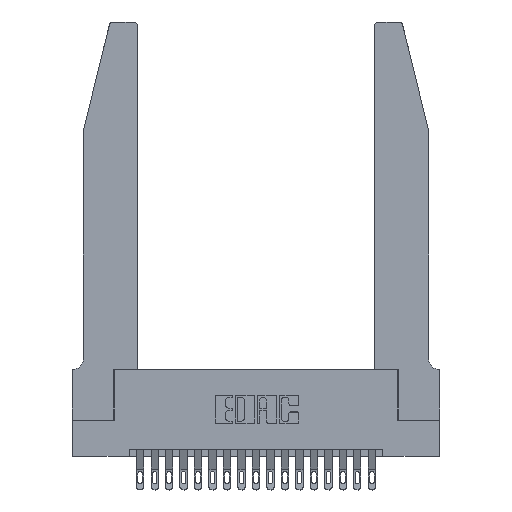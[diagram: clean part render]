
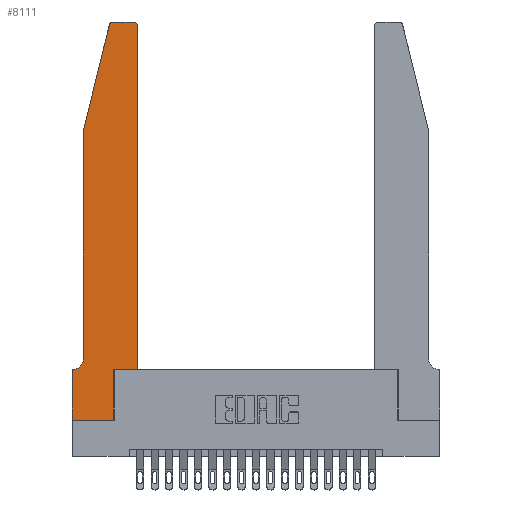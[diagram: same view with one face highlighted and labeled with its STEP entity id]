
A CAD part, top view. The second image highlights one B-rep face of the part: STEP entity #8111.
In plain terms, the highlighted planar face has unit normal (0, 0, 1).
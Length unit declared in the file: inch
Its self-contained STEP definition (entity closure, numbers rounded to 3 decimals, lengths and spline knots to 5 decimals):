
#135 = ORIENTED_EDGE ( 'NONE', *, *, #18145, .T. ) ;
#335 = VERTEX_POINT ( 'NONE', #13361 ) ;
#349 = CARTESIAN_POINT ( 'NONE',  ( 0.4205, 2.72, 0.37 ) ) ;
#358 = DIRECTION ( 'NONE',  ( 0., 0., 1. ) ) ;
#397 = CARTESIAN_POINT ( 'NONE',  ( 0.2605, 2.75, 0.37 ) ) ;
#501 = DIRECTION ( 'NONE',  ( 0., 0., 1. ) ) ;
#661 = DIRECTION ( 'NONE',  ( 1., 0., 0. ) ) ;
#810 = CARTESIAN_POINT ( 'NONE',  ( 0.0755, 0.35, 0.37 ) ) ;
#831 = EDGE_CURVE ( 'NONE', #11296, #10545, #4800, .T. ) ;
#988 = CIRCLE ( 'NONE', #9246, 0.03 ) ;
#994 = EDGE_CURVE ( 'NONE', #17987, #8343, #1332, .T. ) ;
#1332 = LINE ( 'NONE', #8195, #12391 ) ;
#1522 = VERTEX_POINT ( 'NONE', #14327 ) ;
#1997 = VERTEX_POINT ( 'NONE', #9547 ) ;
#2032 = DIRECTION ( 'NONE',  ( 1., 0., 0. ) ) ;
#2087 = DIRECTION ( 'NONE',  ( -1., 0., 0. ) ) ;
#2121 = VECTOR ( 'NONE', #18065, 39.37008 ) ;
#2178 = VERTEX_POINT ( 'NONE', #17374 ) ;
#2196 = DIRECTION ( 'NONE',  ( 1., 0., 0. ) ) ;
#2197 = CARTESIAN_POINT ( 'NONE',  ( 0.284, 2.72, 0.37 ) ) ;
#2443 = CARTESIAN_POINT ( 'NONE',  ( 0.4505, 0.35, 0.37 ) ) ;
#2599 = CIRCLE ( 'NONE', #20551, 0.07 ) ;
#2763 = CARTESIAN_POINT ( 'NONE',  ( 0.2865, 0.35, 0.37 ) ) ;
#2935 = DIRECTION ( 'NONE',  ( 0., 1., 0. ) ) ;
#3291 = FACE_OUTER_BOUND ( 'NONE', #15871, .T. ) ;
#4286 = VECTOR ( 'NONE', #5819, 39.37008 ) ;
#4567 = VECTOR ( 'NONE', #661, 39.37008 ) ;
#4800 = LINE ( 'NONE', #2763, #2121 ) ;
#4857 = LINE ( 'NONE', #397, #12748 ) ;
#5289 = CARTESIAN_POINT ( 'NONE',  ( 0.0755, 2., 0.37 ) ) ;
#5392 = LINE ( 'NONE', #17648, #11170 ) ;
#5469 = EDGE_CURVE ( 'NONE', #7571, #12165, #5392, .T. ) ;
#5819 = DIRECTION ( 'NONE',  ( -1., 0., 0. ) ) ;
#5886 = ORIENTED_EDGE ( 'NONE', *, *, #18480, .T. ) ;
#6078 = ORIENTED_EDGE ( 'NONE', *, *, #10232, .T. ) ;
#6089 = EDGE_CURVE ( 'NONE', #10545, #1997, #9056, .T. ) ;
#7118 = CARTESIAN_POINT ( 'NONE',  ( 0., 0.35, 0.37 ) ) ;
#7571 = VERTEX_POINT ( 'NONE', #20167 ) ;
#7672 = CARTESIAN_POINT ( 'NONE',  ( 0.0055, 0.42, 0.37 ) ) ;
#7770 = DIRECTION ( 'NONE',  ( 0., -1., 0. ) ) ;
#7857 = CARTESIAN_POINT ( 'NONE',  ( 0.4505, 0.35, 0.37 ) ) ;
#8111 = ADVANCED_FACE ( 'NONE', ( #3291 ), #10648, .T. ) ;
#8195 = CARTESIAN_POINT ( 'NONE',  ( 0.0755, 2., 0.37 ) ) ;
#8343 = VERTEX_POINT ( 'NONE', #5289 ) ;
#8538 = EDGE_CURVE ( 'NONE', #335, #17987, #12736, .T. ) ;
#8607 = VECTOR ( 'NONE', #2935, 39.37008 ) ;
#9056 = LINE ( 'NONE', #2443, #4567 ) ;
#9246 = AXIS2_PLACEMENT_3D ( 'NONE', #349, #501, #2196 ) ;
#9290 = EDGE_CURVE ( 'NONE', #12315, #7571, #16645, .T. ) ;
#9384 = DIRECTION ( 'NONE',  ( -1., 0., 0. ) ) ;
#9547 = CARTESIAN_POINT ( 'NONE',  ( 0.4505, 0.35, 0.37 ) ) ;
#10099 = DIRECTION ( 'NONE',  ( -0.239, -0.971, 0. ) ) ;
#10232 = EDGE_CURVE ( 'NONE', #8343, #1522, #16864, .T. ) ;
#10334 = ORIENTED_EDGE ( 'NONE', *, *, #831, .T. ) ;
#10497 = ORIENTED_EDGE ( 'NONE', *, *, #17471, .T. ) ;
#10545 = VERTEX_POINT ( 'NONE', #18705 ) ;
#10648 = PLANE ( 'NONE',  #12534 ) ;
#11127 = CARTESIAN_POINT ( 'NONE',  ( 0., 0., 0.37 ) ) ;
#11170 = VECTOR ( 'NONE', #7770, 39.37008 ) ;
#11296 = VERTEX_POINT ( 'NONE', #20777 ) ;
#11464 = ORIENTED_EDGE ( 'NONE', *, *, #5469, .T. ) ;
#11802 = VECTOR ( 'NONE', #2032, 39.37008 ) ;
#12165 = VERTEX_POINT ( 'NONE', #11127 ) ;
#12201 = CARTESIAN_POINT ( 'NONE',  ( 0.0055, 0.35, 0.37 ) ) ;
#12205 = DIRECTION ( 'NONE',  ( 0., 0., 1. ) ) ;
#12315 = VERTEX_POINT ( 'NONE', #12201 ) ;
#12319 = LINE ( 'NONE', #12341, #11802 ) ;
#12341 = CARTESIAN_POINT ( 'NONE',  ( 0., 0., 0.37 ) ) ;
#12343 = CARTESIAN_POINT ( 'NONE',  ( 0.4205, 2.75, 0.37 ) ) ;
#12389 = AXIS2_PLACEMENT_3D ( 'NONE', #2197, #12205, #13972 ) ;
#12391 = VECTOR ( 'NONE', #10099, 39.37008 ) ;
#12461 = VERTEX_POINT ( 'NONE', #12343 ) ;
#12534 = AXIS2_PLACEMENT_3D ( 'NONE', #7118, #358, #18776 ) ;
#12736 = CIRCLE ( 'NONE', #12389, 0.03 ) ;
#12748 = VECTOR ( 'NONE', #2087, 39.37008 ) ;
#13354 = ORIENTED_EDGE ( 'NONE', *, *, #6089, .T. ) ;
#13361 = CARTESIAN_POINT ( 'NONE',  ( 0.284, 2.75, 0.37 ) ) ;
#13422 = ORIENTED_EDGE ( 'NONE', *, *, #19981, .T. ) ;
#13972 = DIRECTION ( 'NONE',  ( 1., 0., 0. ) ) ;
#14318 = CARTESIAN_POINT ( 'NONE',  ( 0.0755, 2., 0.37 ) ) ;
#14327 = CARTESIAN_POINT ( 'NONE',  ( 0.0755, 0.42, 0.37 ) ) ;
#14793 = EDGE_CURVE ( 'NONE', #12461, #335, #4857, .T. ) ;
#14843 = ORIENTED_EDGE ( 'NONE', *, *, #994, .T. ) ;
#15308 = ORIENTED_EDGE ( 'NONE', *, *, #9290, .T. ) ;
#15773 = DIRECTION ( 'NONE',  ( 0., -1., 0. ) ) ;
#15871 = EDGE_LOOP ( 'NONE', ( #17800, #18323, #14843, #6078, #10497, #15308, #11464, #135, #10334, #13354, #5886, #13422 ) ) ;
#16645 = LINE ( 'NONE', #810, #4286 ) ;
#16864 = LINE ( 'NONE', #14318, #17393 ) ;
#16922 = CARTESIAN_POINT ( 'NONE',  ( 0.25487, 2.72718, 0.37 ) ) ;
#17374 = CARTESIAN_POINT ( 'NONE',  ( 0.4505, 2.72, 0.37 ) ) ;
#17393 = VECTOR ( 'NONE', #15773, 39.37008 ) ;
#17471 = EDGE_CURVE ( 'NONE', #1522, #12315, #2599, .T. ) ;
#17580 = LINE ( 'NONE', #7857, #8607 ) ;
#17648 = CARTESIAN_POINT ( 'NONE',  ( 0., 0., 0.37 ) ) ;
#17800 = ORIENTED_EDGE ( 'NONE', *, *, #14793, .T. ) ;
#17987 = VERTEX_POINT ( 'NONE', #16922 ) ;
#18065 = DIRECTION ( 'NONE',  ( 0., 1., 0. ) ) ;
#18145 = EDGE_CURVE ( 'NONE', #12165, #11296, #12319, .T. ) ;
#18323 = ORIENTED_EDGE ( 'NONE', *, *, #8538, .T. ) ;
#18480 = EDGE_CURVE ( 'NONE', #1997, #2178, #17580, .T. ) ;
#18705 = CARTESIAN_POINT ( 'NONE',  ( 0.2865, 0.35, 0.37 ) ) ;
#18776 = DIRECTION ( 'NONE',  ( 1., 0., 0. ) ) ;
#19443 = DIRECTION ( 'NONE',  ( 0., 0., -1. ) ) ;
#19981 = EDGE_CURVE ( 'NONE', #2178, #12461, #988, .T. ) ;
#20167 = CARTESIAN_POINT ( 'NONE',  ( 0., 0.35, 0.37 ) ) ;
#20551 = AXIS2_PLACEMENT_3D ( 'NONE', #7672, #19443, #9384 ) ;
#20777 = CARTESIAN_POINT ( 'NONE',  ( 0.2865, 0., 0.37 ) ) ;
